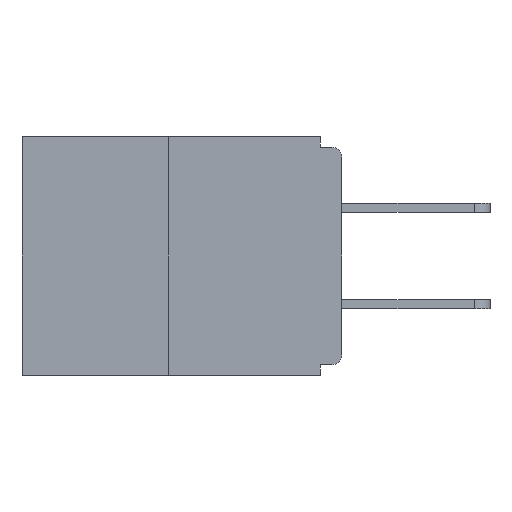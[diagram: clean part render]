
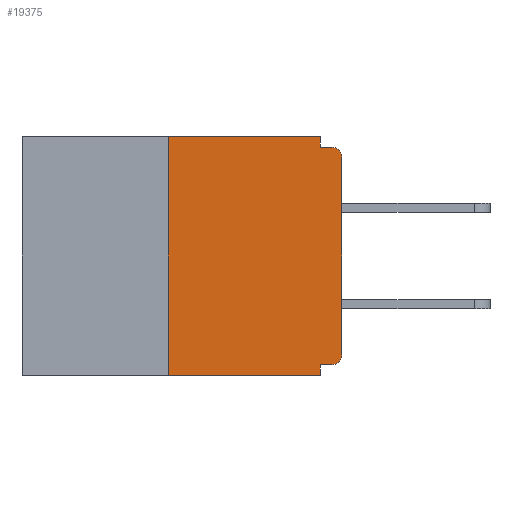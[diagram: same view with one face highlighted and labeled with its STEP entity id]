
A CAD part, left-side view. The second image highlights one B-rep face of the part: STEP entity #19375.
In plain terms, the highlighted planar face has unit normal (-1, 0, 0).
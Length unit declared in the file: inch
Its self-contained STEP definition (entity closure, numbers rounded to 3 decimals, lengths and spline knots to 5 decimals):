
#73 = CARTESIAN_POINT ( 'NONE',  ( 0., 0., 0. ) ) ;
#239 = DIRECTION ( 'NONE',  ( 0., 0., -1. ) ) ;
#394 = DIRECTION ( 'NONE',  ( 0., 0., 1. ) ) ;
#1588 = CARTESIAN_POINT ( 'NONE',  ( 0., 0., -0.313 ) ) ;
#1693 = ORIENTED_EDGE ( 'NONE', *, *, #21767, .T. ) ;
#1971 = EDGE_CURVE ( 'NONE', #26724, #19283, #22375, .T. ) ;
#2413 = EDGE_CURVE ( 'NONE', #19217, #15219, #22702, .T. ) ;
#2439 = VECTOR ( 'NONE', #3914, 39.37008 ) ;
#2797 = EDGE_CURVE ( 'NONE', #19283, #4896, #14676, .T. ) ;
#3245 = EDGE_CURVE ( 'NONE', #17108, #26042, #10018, .T. ) ;
#3465 = EDGE_CURVE ( 'NONE', #25956, #26042, #11386, .T. ) ;
#3490 = EDGE_LOOP ( 'NONE', ( #12877, #13103, #22521, #14179, #18137, #1693, #7836, #3979, #24779, #24620 ) ) ;
#3702 = VECTOR ( 'NONE', #6942, 39.37008 ) ;
#3914 = DIRECTION ( 'NONE',  ( 0., -1., 0. ) ) ;
#3979 = ORIENTED_EDGE ( 'NONE', *, *, #2413, .T. ) ;
#4705 = DIRECTION ( 'NONE',  ( 0., 0., 1. ) ) ;
#4896 = VERTEX_POINT ( 'NONE', #6602 ) ;
#5174 = DIRECTION ( 'NONE',  ( 1., 0., 0. ) ) ;
#5435 = CARTESIAN_POINT ( 'NONE',  ( 0., 0.46, 0. ) ) ;
#5694 = VECTOR ( 'NONE', #6250, 39.37008 ) ;
#6250 = DIRECTION ( 'NONE',  ( 0., -1., 0. ) ) ;
#6307 = VERTEX_POINT ( 'NONE', #1588 ) ;
#6528 = LINE ( 'NONE', #18186, #14821 ) ;
#6602 = CARTESIAN_POINT ( 'NONE',  ( 0., 0.031, -0.015 ) ) ;
#6614 = DIRECTION ( 'NONE',  ( 0., 0., -1. ) ) ;
#6622 = DIRECTION ( 'NONE',  ( -1., 0., 0. ) ) ;
#6942 = DIRECTION ( 'NONE',  ( 0., 0., -1. ) ) ;
#7133 = CARTESIAN_POINT ( 'NONE',  ( 0., 0., -0.03 ) ) ;
#7665 = PLANE ( 'NONE',  #9910 ) ;
#7836 = ORIENTED_EDGE ( 'NONE', *, *, #26416, .T. ) ;
#8302 = CARTESIAN_POINT ( 'NONE',  ( 0., 0.46, -0.343 ) ) ;
#8358 = VECTOR ( 'NONE', #18602, 39.37008 ) ;
#8847 = CARTESIAN_POINT ( 'NONE',  ( 0., 0.031, -0.343 ) ) ;
#9075 = CARTESIAN_POINT ( 'NONE',  ( 0., 0.031, 0. ) ) ;
#9522 = DIRECTION ( 'NONE',  ( 0., 0., -1. ) ) ;
#9910 = AXIS2_PLACEMENT_3D ( 'NONE', #5435, #5174, #9522 ) ;
#10018 = LINE ( 'NONE', #8847, #25685 ) ;
#10031 = CARTESIAN_POINT ( 'NONE',  ( 0., 0.015, -0.03 ) ) ;
#10938 = VECTOR ( 'NONE', #4705, 39.37008 ) ;
#11257 = LINE ( 'NONE', #73, #10938 ) ;
#11386 = LINE ( 'NONE', #8302, #5694 ) ;
#12373 = DIRECTION ( 'NONE',  ( -1., 0., 0. ) ) ;
#12655 = FACE_OUTER_BOUND ( 'NONE', #3490, .T. ) ;
#12877 = ORIENTED_EDGE ( 'NONE', *, *, #1971, .F. ) ;
#12995 = CARTESIAN_POINT ( 'NONE',  ( 0., 0.25, -0.343 ) ) ;
#13103 = ORIENTED_EDGE ( 'NONE', *, *, #14701, .F. ) ;
#14179 = ORIENTED_EDGE ( 'NONE', *, *, #3245, .F. ) ;
#14340 = VECTOR ( 'NONE', #394, 39.37008 ) ;
#14676 = LINE ( 'NONE', #9075, #3702 ) ;
#14701 = EDGE_CURVE ( 'NONE', #25956, #26724, #17329, .T. ) ;
#14821 = VECTOR ( 'NONE', #26576, 39.37008 ) ;
#15219 = VERTEX_POINT ( 'NONE', #16292 ) ;
#15738 = CARTESIAN_POINT ( 'NONE',  ( 0., 0.015, -0.328 ) ) ;
#16292 = CARTESIAN_POINT ( 'NONE',  ( 0., 0.015, -0.015 ) ) ;
#16566 = CARTESIAN_POINT ( 'NONE',  ( 0., 0.25, 0. ) ) ;
#16896 = CARTESIAN_POINT ( 'NONE',  ( 0., 0.46, 0. ) ) ;
#17108 = VERTEX_POINT ( 'NONE', #21380 ) ;
#17329 = LINE ( 'NONE', #23512, #14340 ) ;
#17589 = CARTESIAN_POINT ( 'NONE',  ( 0., 0.031, 0. ) ) ;
#17759 = AXIS2_PLACEMENT_3D ( 'NONE', #10031, #12373, #24923 ) ;
#18137 = ORIENTED_EDGE ( 'NONE', *, *, #27280, .F. ) ;
#18186 = CARTESIAN_POINT ( 'NONE',  ( 0., 0., -0.328 ) ) ;
#18602 = DIRECTION ( 'NONE',  ( 0., -1., 0. ) ) ;
#18752 = CIRCLE ( 'NONE', #19010, 0.015 ) ;
#19010 = AXIS2_PLACEMENT_3D ( 'NONE', #21694, #6622, #239 ) ;
#19217 = VERTEX_POINT ( 'NONE', #7133 ) ;
#19283 = VERTEX_POINT ( 'NONE', #17589 ) ;
#19375 = ADVANCED_FACE ( 'NONE', ( #12655 ), #7665, .F. ) ;
#19427 = CARTESIAN_POINT ( 'NONE',  ( 0., 0.031, -0.343 ) ) ;
#21380 = CARTESIAN_POINT ( 'NONE',  ( 0., 0.031, -0.328 ) ) ;
#21694 = CARTESIAN_POINT ( 'NONE',  ( 0., 0.015, -0.313 ) ) ;
#21767 = EDGE_CURVE ( 'NONE', #23982, #6307, #18752, .T. ) ;
#22333 = LINE ( 'NONE', #27170, #8358 ) ;
#22375 = LINE ( 'NONE', #16896, #2439 ) ;
#22521 = ORIENTED_EDGE ( 'NONE', *, *, #3465, .T. ) ;
#22702 = CIRCLE ( 'NONE', #17759, 0.015 ) ;
#23512 = CARTESIAN_POINT ( 'NONE',  ( 0., 0.25, 0. ) ) ;
#23982 = VERTEX_POINT ( 'NONE', #15738 ) ;
#24221 = EDGE_CURVE ( 'NONE', #4896, #15219, #22333, .T. ) ;
#24620 = ORIENTED_EDGE ( 'NONE', *, *, #2797, .F. ) ;
#24779 = ORIENTED_EDGE ( 'NONE', *, *, #24221, .F. ) ;
#24923 = DIRECTION ( 'NONE',  ( 0., 0., -1. ) ) ;
#25685 = VECTOR ( 'NONE', #6614, 39.37008 ) ;
#25956 = VERTEX_POINT ( 'NONE', #12995 ) ;
#26042 = VERTEX_POINT ( 'NONE', #19427 ) ;
#26416 = EDGE_CURVE ( 'NONE', #6307, #19217, #11257, .T. ) ;
#26576 = DIRECTION ( 'NONE',  ( 0., 1., 0. ) ) ;
#26724 = VERTEX_POINT ( 'NONE', #16566 ) ;
#27170 = CARTESIAN_POINT ( 'NONE',  ( 0., 0., -0.015 ) ) ;
#27280 = EDGE_CURVE ( 'NONE', #23982, #17108, #6528, .T. ) ;
